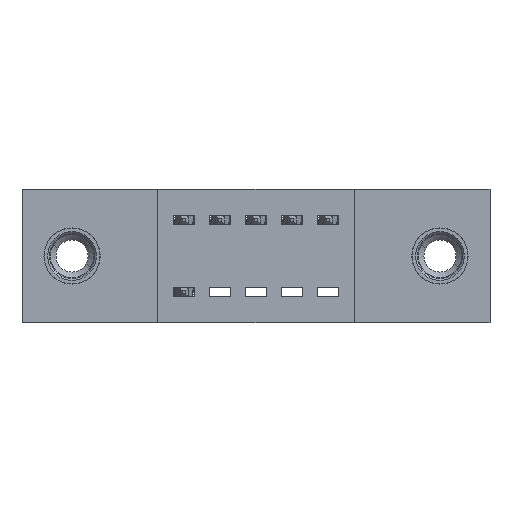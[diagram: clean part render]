
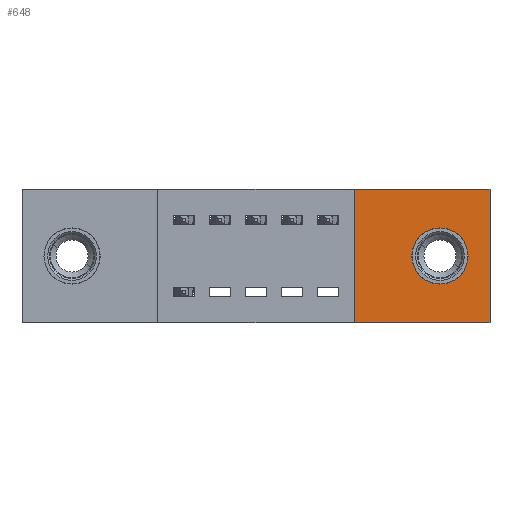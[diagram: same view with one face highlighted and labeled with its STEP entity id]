
A CAD part, front view. The second image highlights one B-rep face of the part: STEP entity #648.
In plain terms, the highlighted planar face has unit normal (0, -1, 0).
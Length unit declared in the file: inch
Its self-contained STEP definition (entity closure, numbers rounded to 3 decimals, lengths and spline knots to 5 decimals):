
#82 = ORIENTED_EDGE ( 'NONE', *, *, #795, .T. ) ;
#101 = VERTEX_POINT ( 'NONE', #1970 ) ;
#134 = EDGE_LOOP ( 'NONE', ( #1441, #82 ) ) ;
#439 = DIRECTION ( 'NONE',  ( 0., 1., 0. ) ) ;
#646 = DIRECTION ( 'NONE',  ( -1., 0., 0. ) ) ;
#648 = ADVANCED_FACE ( 'NONE', ( #7656, #4265 ), #3880, .T. ) ;
#696 = CARTESIAN_POINT ( 'NONE',  ( 1.161, 0., -0.185 ) ) ;
#795 = EDGE_CURVE ( 'NONE', #6876, #4275, #4787, .T. ) ;
#895 = DIRECTION ( 'NONE',  ( 0., 0., -1. ) ) ;
#983 = LINE ( 'NONE', #5306, #3110 ) ;
#1115 = DIRECTION ( 'NONE',  ( 1., 0., 0. ) ) ;
#1238 = VECTOR ( 'NONE', #1837, 39.37008 ) ;
#1385 = DIRECTION ( 'NONE',  ( 0., 0., -1. ) ) ;
#1441 = ORIENTED_EDGE ( 'NONE', *, *, #1610, .T. ) ;
#1610 = EDGE_CURVE ( 'NONE', #4275, #6876, #1967, .T. ) ;
#1833 = LINE ( 'NONE', #2119, #7111 ) ;
#1837 = DIRECTION ( 'NONE',  ( 0., 0., 1. ) ) ;
#1909 = CARTESIAN_POINT ( 'NONE',  ( 0.923, 0., 0. ) ) ;
#1967 = CIRCLE ( 'NONE', #5156, 0.078 ) ;
#1970 = CARTESIAN_POINT ( 'NONE',  ( 1.3, 0., -0.37 ) ) ;
#2025 = ORIENTED_EDGE ( 'NONE', *, *, #2357, .F. ) ;
#2119 = CARTESIAN_POINT ( 'NONE',  ( 0., 0., -0.37 ) ) ;
#2239 = CARTESIAN_POINT ( 'NONE',  ( 1.161, 0., -0.185 ) ) ;
#2357 = EDGE_CURVE ( 'NONE', #101, #2691, #1833, .T. ) ;
#2424 = DIRECTION ( 'NONE',  ( 0., 0., -1. ) ) ;
#2643 = EDGE_CURVE ( 'NONE', #2691, #8648, #6804, .T. ) ;
#2691 = VERTEX_POINT ( 'NONE', #8645 ) ;
#2723 = DIRECTION ( 'NONE',  ( 0., 1., 0. ) ) ;
#2823 = CARTESIAN_POINT ( 'NONE',  ( 0., 0., -0.37 ) ) ;
#3110 = VECTOR ( 'NONE', #1115, 39.37008 ) ;
#3375 = CARTESIAN_POINT ( 'NONE',  ( 1.161, 0., -0.107 ) ) ;
#3501 = EDGE_CURVE ( 'NONE', #8648, #3651, #983, .T. ) ;
#3651 = VERTEX_POINT ( 'NONE', #4767 ) ;
#3754 = EDGE_CURVE ( 'NONE', #3651, #101, #4398, .T. ) ;
#3880 = PLANE ( 'NONE',  #6125 ) ;
#3975 = DIRECTION ( 'NONE',  ( 0., 0., -1. ) ) ;
#4175 = EDGE_LOOP ( 'NONE', ( #8838, #2025, #7482, #8120 ) ) ;
#4265 = FACE_OUTER_BOUND ( 'NONE', #4175, .T. ) ;
#4275 = VERTEX_POINT ( 'NONE', #3375 ) ;
#4326 = DIRECTION ( 'NONE',  ( 0., -1., 0. ) ) ;
#4398 = LINE ( 'NONE', #5562, #8211 ) ;
#4767 = CARTESIAN_POINT ( 'NONE',  ( 1.3, 0., 0. ) ) ;
#4787 = CIRCLE ( 'NONE', #7935, 0.078 ) ;
#5156 = AXIS2_PLACEMENT_3D ( 'NONE', #2239, #2723, #895 ) ;
#5306 = CARTESIAN_POINT ( 'NONE',  ( 0., 0., 0. ) ) ;
#5562 = CARTESIAN_POINT ( 'NONE',  ( 1.3, 0., 0. ) ) ;
#6125 = AXIS2_PLACEMENT_3D ( 'NONE', #2823, #4326, #3975 ) ;
#6804 = LINE ( 'NONE', #8383, #1238 ) ;
#6869 = CARTESIAN_POINT ( 'NONE',  ( 1.161, 0., -0.263 ) ) ;
#6876 = VERTEX_POINT ( 'NONE', #6869 ) ;
#7111 = VECTOR ( 'NONE', #646, 39.37008 ) ;
#7482 = ORIENTED_EDGE ( 'NONE', *, *, #3754, .F. ) ;
#7656 = FACE_BOUND ( 'NONE', #134, .T. ) ;
#7935 = AXIS2_PLACEMENT_3D ( 'NONE', #696, #439, #2424 ) ;
#8120 = ORIENTED_EDGE ( 'NONE', *, *, #3501, .F. ) ;
#8211 = VECTOR ( 'NONE', #1385, 39.37008 ) ;
#8383 = CARTESIAN_POINT ( 'NONE',  ( 0.923, 0., -0.37 ) ) ;
#8645 = CARTESIAN_POINT ( 'NONE',  ( 0.923, 0., -0.37 ) ) ;
#8648 = VERTEX_POINT ( 'NONE', #1909 ) ;
#8838 = ORIENTED_EDGE ( 'NONE', *, *, #2643, .F. ) ;
